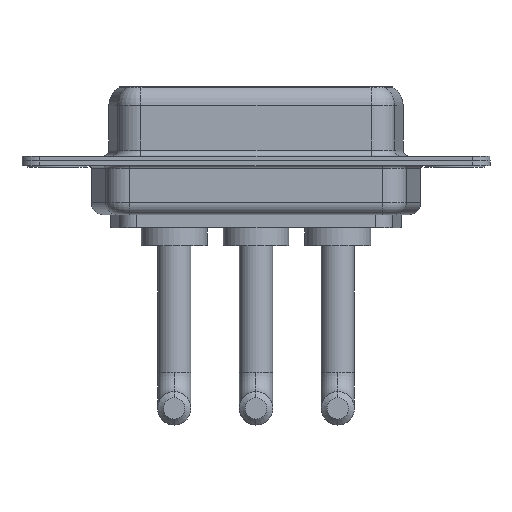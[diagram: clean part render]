
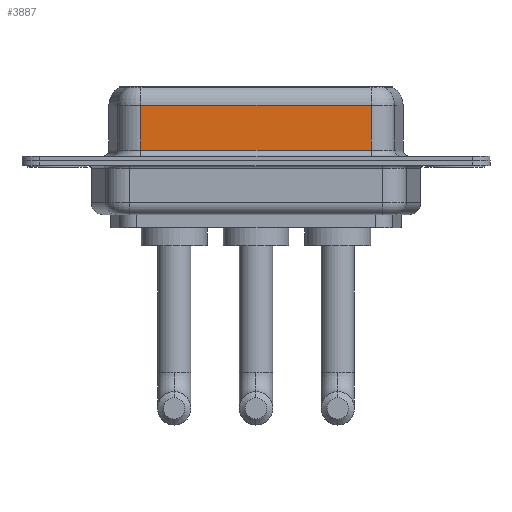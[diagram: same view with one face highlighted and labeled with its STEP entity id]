
A CAD part, front view. The second image highlights one B-rep face of the part: STEP entity #3887.
In plain terms, the highlighted planar face has unit normal (0, -1, 0).
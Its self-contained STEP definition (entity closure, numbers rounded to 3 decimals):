
#27 = LINE ( 'NONE', #7514, #9763 ) ;
#475 = CARTESIAN_POINT ( 'NONE',  ( 7.013, -3.95, 0.9 ) ) ;
#631 = EDGE_CURVE ( 'NONE', #5403, #4151, #27, .T. ) ;
#806 = EDGE_CURVE ( 'NONE', #4392, #2490, #4350, .T. ) ;
#1206 = DIRECTION ( 'NONE',  ( 0., 0., -1. ) ) ;
#1341 = CARTESIAN_POINT ( 'NONE',  ( 26.287, -3.95, 0.9 ) ) ;
#1501 = ORIENTED_EDGE ( 'NONE', *, *, #631, .F. ) ;
#1956 = CARTESIAN_POINT ( 'NONE',  ( 7.013, -3.95, 6.4 ) ) ;
#2025 = CARTESIAN_POINT ( 'NONE',  ( 26.287, -3.95, 4.65 ) ) ;
#2078 = ORIENTED_EDGE ( 'NONE', *, *, #4399, .T. ) ;
#2095 = CARTESIAN_POINT ( 'NONE',  ( 26.287, -3.95, 6.4 ) ) ;
#2490 = VERTEX_POINT ( 'NONE', #475 ) ;
#2520 = CARTESIAN_POINT ( 'NONE',  ( 26.287, -3.95, 0.9 ) ) ;
#2530 = EDGE_CURVE ( 'NONE', #2490, #4151, #6146, .T. ) ;
#2554 = ORIENTED_EDGE ( 'NONE', *, *, #2530, .T. ) ;
#2586 = ORIENTED_EDGE ( 'NONE', *, *, #806, .T. ) ;
#2835 = CARTESIAN_POINT ( 'NONE',  ( 7.013, -3.95, 4.65 ) ) ;
#2890 = DIRECTION ( 'NONE',  ( 1., 0., 0. ) ) ;
#3524 = EDGE_LOOP ( 'NONE', ( #1501, #2078, #2586, #2554 ) ) ;
#3575 = DIRECTION ( 'NONE',  ( -1., 0., 0. ) ) ;
#3680 = LINE ( 'NONE', #2025, #9055 ) ;
#3887 = ADVANCED_FACE ( 'NONE', ( #10261 ), #6149, .F. ) ;
#4151 = VERTEX_POINT ( 'NONE', #2520 ) ;
#4350 = LINE ( 'NONE', #1956, #7550 ) ;
#4392 = VERTEX_POINT ( 'NONE', #2835 ) ;
#4399 = EDGE_CURVE ( 'NONE', #5403, #4392, #3680, .T. ) ;
#4497 = DIRECTION ( 'NONE',  ( 0., 0., 1. ) ) ;
#4946 = AXIS2_PLACEMENT_3D ( 'NONE', #2095, #10168, #4497 ) ;
#5403 = VERTEX_POINT ( 'NONE', #5587 ) ;
#5587 = CARTESIAN_POINT ( 'NONE',  ( 26.287, -3.95, 4.65 ) ) ;
#6146 = LINE ( 'NONE', #1341, #9052 ) ;
#6149 = PLANE ( 'NONE',  #4946 ) ;
#7514 = CARTESIAN_POINT ( 'NONE',  ( 26.287, -3.95, 6.4 ) ) ;
#7550 = VECTOR ( 'NONE', #1206, 1000. ) ;
#9052 = VECTOR ( 'NONE', #2890, 1000. ) ;
#9055 = VECTOR ( 'NONE', #3575, 1000. ) ;
#9763 = VECTOR ( 'NONE', #9815, 1000. ) ;
#9815 = DIRECTION ( 'NONE',  ( 0., 0., -1. ) ) ;
#10168 = DIRECTION ( 'NONE',  ( 0., 1., 0. ) ) ;
#10261 = FACE_OUTER_BOUND ( 'NONE', #3524, .T. ) ;
